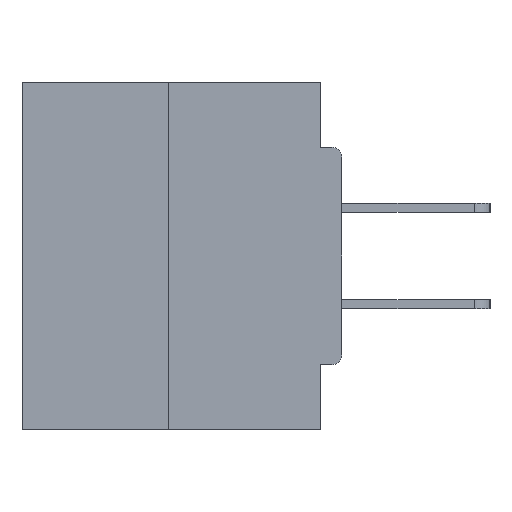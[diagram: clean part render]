
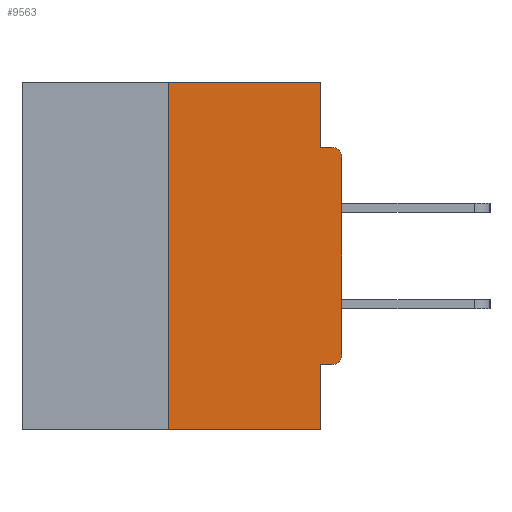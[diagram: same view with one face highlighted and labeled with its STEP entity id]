
A CAD part, left-side view. The second image highlights one B-rep face of the part: STEP entity #9563.
In plain terms, the highlighted planar face has unit normal (-1, 0, 0).
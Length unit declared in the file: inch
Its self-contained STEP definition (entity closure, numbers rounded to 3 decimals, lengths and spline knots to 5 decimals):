
#510 = VERTEX_POINT ( 'NONE', #4629 ) ;
#533 = AXIS2_PLACEMENT_3D ( 'NONE', #21833, #19381, #8920 ) ;
#686 = EDGE_CURVE ( 'NONE', #30449, #16919, #7037, .T. ) ;
#1237 = ORIENTED_EDGE ( 'NONE', *, *, #32731, .T. ) ;
#2137 = CARTESIAN_POINT ( 'NONE',  ( 0., 0.46, 0. ) ) ;
#2868 = VECTOR ( 'NONE', #18756, 39.37008 ) ;
#3388 = ORIENTED_EDGE ( 'NONE', *, *, #17783, .F. ) ;
#4196 = ORIENTED_EDGE ( 'NONE', *, *, #29894, .T. ) ;
#4461 = CARTESIAN_POINT ( 'NONE',  ( 0., 0., 0. ) ) ;
#4629 = CARTESIAN_POINT ( 'NONE',  ( 0., 0.031, -0.0935 ) ) ;
#4950 = DIRECTION ( 'NONE',  ( -1., 0., 0. ) ) ;
#5308 = VECTOR ( 'NONE', #20307, 39.37008 ) ;
#5663 = DIRECTION ( 'NONE',  ( 0., 0., -1. ) ) ;
#5849 = EDGE_CURVE ( 'NONE', #15514, #16210, #29212, .T. ) ;
#6429 = EDGE_CURVE ( 'NONE', #20969, #7975, #29170, .T. ) ;
#7037 = LINE ( 'NONE', #27294, #14687 ) ;
#7975 = VERTEX_POINT ( 'NONE', #22138 ) ;
#8166 = CARTESIAN_POINT ( 'NONE',  ( 0., 0.015, -0.0935 ) ) ;
#8167 = ORIENTED_EDGE ( 'NONE', *, *, #686, .F. ) ;
#8199 = ORIENTED_EDGE ( 'NONE', *, *, #33019, .F. ) ;
#8783 = CARTESIAN_POINT ( 'NONE',  ( 0., 0., -0.0935 ) ) ;
#8920 = DIRECTION ( 'NONE',  ( 0., 0., -1. ) ) ;
#8983 = VECTOR ( 'NONE', #22034, 39.37008 ) ;
#9319 = CARTESIAN_POINT ( 'NONE',  ( 0., 0.031, -0.4065 ) ) ;
#9563 = ADVANCED_FACE ( 'NONE', ( #14559 ), #20004, .F. ) ;
#9656 = EDGE_LOOP ( 'NONE', ( #8167, #8199, #1237, #17502, #16226, #23134, #4196, #26789, #30414, #3388 ) ) ;
#10086 = EDGE_CURVE ( 'NONE', #15514, #20969, #23750, .T. ) ;
#10131 = AXIS2_PLACEMENT_3D ( 'NONE', #25576, #4950, #25362 ) ;
#10144 = EDGE_CURVE ( 'NONE', #510, #16824, #20555, .T. ) ;
#10183 = VERTEX_POINT ( 'NONE', #17568 ) ;
#10505 = LINE ( 'NONE', #27003, #5308 ) ;
#10851 = VERTEX_POINT ( 'NONE', #19052 ) ;
#11498 = DIRECTION ( 'NONE',  ( 0., 0., 1. ) ) ;
#13581 = AXIS2_PLACEMENT_3D ( 'NONE', #2137, #15177, #32896 ) ;
#13610 = CIRCLE ( 'NONE', #10131, 0.015 ) ;
#14559 = FACE_OUTER_BOUND ( 'NONE', #9656, .T. ) ;
#14687 = VECTOR ( 'NONE', #27188, 39.37008 ) ;
#15177 = DIRECTION ( 'NONE',  ( 1., 0., 0. ) ) ;
#15514 = VERTEX_POINT ( 'NONE', #29297 ) ;
#16210 = VERTEX_POINT ( 'NONE', #24614 ) ;
#16226 = ORIENTED_EDGE ( 'NONE', *, *, #10086, .F. ) ;
#16824 = VERTEX_POINT ( 'NONE', #8166 ) ;
#16919 = VERTEX_POINT ( 'NONE', #20619 ) ;
#17502 = ORIENTED_EDGE ( 'NONE', *, *, #6429, .F. ) ;
#17568 = CARTESIAN_POINT ( 'NONE',  ( 0., 0., -0.1085 ) ) ;
#17783 = EDGE_CURVE ( 'NONE', #16919, #510, #10505, .T. ) ;
#18756 = DIRECTION ( 'NONE',  ( 0., 1., 0. ) ) ;
#19052 = CARTESIAN_POINT ( 'NONE',  ( 0., 0.25, -0.5 ) ) ;
#19381 = DIRECTION ( 'NONE',  ( -1., 0., 0. ) ) ;
#19742 = VECTOR ( 'NONE', #32213, 39.37008 ) ;
#19936 = EDGE_CURVE ( 'NONE', #10183, #16824, #13610, .T. ) ;
#20004 = PLANE ( 'NONE',  #13581 ) ;
#20307 = DIRECTION ( 'NONE',  ( 0., 0., -1. ) ) ;
#20555 = LINE ( 'NONE', #8783, #19742 ) ;
#20619 = CARTESIAN_POINT ( 'NONE',  ( 0., 0.031, 0. ) ) ;
#20969 = VERTEX_POINT ( 'NONE', #9319 ) ;
#21045 = CARTESIAN_POINT ( 'NONE',  ( 0., 0.031, -0.5 ) ) ;
#21833 = CARTESIAN_POINT ( 'NONE',  ( 0., 0.015, -0.3915 ) ) ;
#22034 = DIRECTION ( 'NONE',  ( 0., -1., 0. ) ) ;
#22138 = CARTESIAN_POINT ( 'NONE',  ( 0., 0.031, -0.5 ) ) ;
#22269 = LINE ( 'NONE', #32109, #8983 ) ;
#22665 = CARTESIAN_POINT ( 'NONE',  ( 0., 0.25, 0. ) ) ;
#22776 = LINE ( 'NONE', #4461, #24729 ) ;
#22856 = DIRECTION ( 'NONE',  ( 0., 0., 1. ) ) ;
#23134 = ORIENTED_EDGE ( 'NONE', *, *, #5849, .T. ) ;
#23750 = LINE ( 'NONE', #29029, #2868 ) ;
#24178 = CARTESIAN_POINT ( 'NONE',  ( 0., 0.25, 0. ) ) ;
#24614 = CARTESIAN_POINT ( 'NONE',  ( 0., 0., -0.3915 ) ) ;
#24729 = VECTOR ( 'NONE', #22856, 39.37008 ) ;
#25362 = DIRECTION ( 'NONE',  ( 0., 0., -1. ) ) ;
#25576 = CARTESIAN_POINT ( 'NONE',  ( 0., 0.015, -0.1085 ) ) ;
#25603 = VECTOR ( 'NONE', #5663, 39.37008 ) ;
#26789 = ORIENTED_EDGE ( 'NONE', *, *, #19936, .T. ) ;
#27003 = CARTESIAN_POINT ( 'NONE',  ( 0., 0.031, 0. ) ) ;
#27188 = DIRECTION ( 'NONE',  ( 0., -1., 0. ) ) ;
#27294 = CARTESIAN_POINT ( 'NONE',  ( 0., 0.46, 0. ) ) ;
#29029 = CARTESIAN_POINT ( 'NONE',  ( 0., 0., -0.4065 ) ) ;
#29170 = LINE ( 'NONE', #21045, #25603 ) ;
#29212 = CIRCLE ( 'NONE', #533, 0.015 ) ;
#29297 = CARTESIAN_POINT ( 'NONE',  ( 0., 0.015, -0.4065 ) ) ;
#29848 = LINE ( 'NONE', #24178, #31002 ) ;
#29894 = EDGE_CURVE ( 'NONE', #16210, #10183, #22776, .T. ) ;
#30414 = ORIENTED_EDGE ( 'NONE', *, *, #10144, .F. ) ;
#30449 = VERTEX_POINT ( 'NONE', #22665 ) ;
#31002 = VECTOR ( 'NONE', #11498, 39.37008 ) ;
#32109 = CARTESIAN_POINT ( 'NONE',  ( 0., 0.46, -0.5 ) ) ;
#32213 = DIRECTION ( 'NONE',  ( 0., -1., 0. ) ) ;
#32731 = EDGE_CURVE ( 'NONE', #10851, #7975, #22269, .T. ) ;
#32896 = DIRECTION ( 'NONE',  ( 0., 0., -1. ) ) ;
#33019 = EDGE_CURVE ( 'NONE', #10851, #30449, #29848, .T. ) ;
